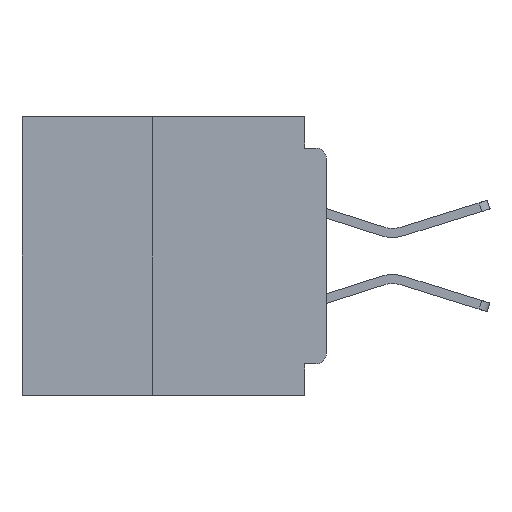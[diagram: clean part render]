
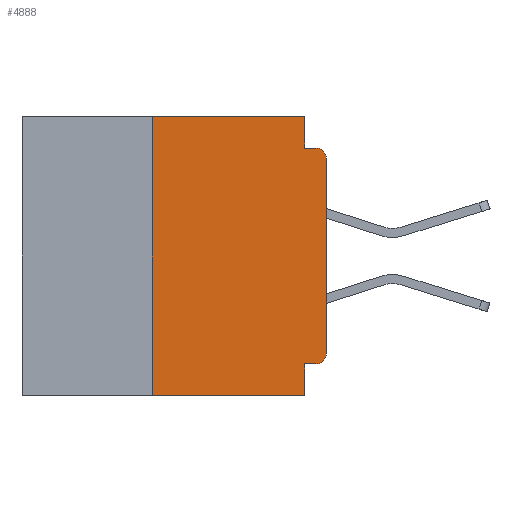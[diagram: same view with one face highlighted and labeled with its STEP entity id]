
A CAD part, left-side view. The second image highlights one B-rep face of the part: STEP entity #4888.
In plain terms, the highlighted planar face has unit normal (-1, 0, 0).
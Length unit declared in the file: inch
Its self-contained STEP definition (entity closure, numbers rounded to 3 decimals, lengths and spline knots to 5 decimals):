
#1334 = ORIENTED_EDGE ( 'NONE', *, *, #21877, .T. ) ;
#1456 = ORIENTED_EDGE ( 'NONE', *, *, #16389, .F. ) ;
#1601 = EDGE_CURVE ( 'NONE', #30420, #3895, #35612, .T. ) ;
#2708 = FACE_OUTER_BOUND ( 'NONE', #19531, .T. ) ;
#3082 = ORIENTED_EDGE ( 'NONE', *, *, #38399, .F. ) ;
#3895 = VERTEX_POINT ( 'NONE', #26321 ) ;
#4888 = ADVANCED_FACE ( 'NONE', ( #2708 ), #45290, .F. ) ;
#5222 = CARTESIAN_POINT ( 'NONE',  ( 0., 0., -0.06 ) ) ;
#5250 = CARTESIAN_POINT ( 'NONE',  ( 0., 0.015, -0.34 ) ) ;
#5289 = EDGE_CURVE ( 'NONE', #10320, #44615, #23680, .T. ) ;
#5556 = VERTEX_POINT ( 'NONE', #16512 ) ;
#5705 = ORIENTED_EDGE ( 'NONE', *, *, #31694, .T. ) ;
#6095 = ORIENTED_EDGE ( 'NONE', *, *, #5289, .F. ) ;
#6575 = CARTESIAN_POINT ( 'NONE',  ( 0., 0.015, -0.355 ) ) ;
#7450 = CARTESIAN_POINT ( 'NONE',  ( 0., 0., -0.045 ) ) ;
#7767 = CARTESIAN_POINT ( 'NONE',  ( 0., 0.25, -0.4 ) ) ;
#8783 = DIRECTION ( 'NONE',  ( 0., 0., -1. ) ) ;
#9641 = VECTOR ( 'NONE', #17980, 39.37008 ) ;
#9995 = LINE ( 'NONE', #41851, #18251 ) ;
#10320 = VERTEX_POINT ( 'NONE', #18087 ) ;
#10326 = DIRECTION ( 'NONE',  ( 0., -1., 0. ) ) ;
#12837 = VECTOR ( 'NONE', #23956, 39.37008 ) ;
#13194 = VERTEX_POINT ( 'NONE', #39578 ) ;
#13732 = EDGE_CURVE ( 'NONE', #3895, #30593, #20109, .T. ) ;
#14413 = CARTESIAN_POINT ( 'NONE',  ( 0., 0.031, -0.4 ) ) ;
#14855 = AXIS2_PLACEMENT_3D ( 'NONE', #44975, #44674, #44639 ) ;
#16389 = EDGE_CURVE ( 'NONE', #18699, #10320, #9995, .T. ) ;
#16512 = CARTESIAN_POINT ( 'NONE',  ( 0., 0.015, -0.045 ) ) ;
#16825 = VECTOR ( 'NONE', #38955, 39.37008 ) ;
#17869 = VERTEX_POINT ( 'NONE', #7767 ) ;
#17980 = DIRECTION ( 'NONE',  ( 0., 0., -1. ) ) ;
#18087 = CARTESIAN_POINT ( 'NONE',  ( 0., 0.031, 0. ) ) ;
#18251 = VECTOR ( 'NONE', #10326, 39.37008 ) ;
#18559 = CIRCLE ( 'NONE', #26442, 0.015 ) ;
#18699 = VERTEX_POINT ( 'NONE', #35764 ) ;
#18898 = EDGE_CURVE ( 'NONE', #30420, #13194, #18559, .T. ) ;
#19531 = EDGE_LOOP ( 'NONE', ( #5705, #1334, #25753, #6095, #1456, #3082, #44940, #28429, #26137, #43435 ) ) ;
#20109 = LINE ( 'NONE', #14413, #9641 ) ;
#20472 = EDGE_CURVE ( 'NONE', #44615, #5556, #40925, .T. ) ;
#20617 = CARTESIAN_POINT ( 'NONE',  ( 0., 0., 0. ) ) ;
#20656 = VECTOR ( 'NONE', #34795, 39.37008 ) ;
#21067 = CARTESIAN_POINT ( 'NONE',  ( 0., 0.015, -0.06 ) ) ;
#21877 = EDGE_CURVE ( 'NONE', #38061, #5556, #42961, .T. ) ;
#22229 = VECTOR ( 'NONE', #38963, 39.37008 ) ;
#23680 = LINE ( 'NONE', #29324, #31943 ) ;
#23802 = LINE ( 'NONE', #45582, #32065 ) ;
#23956 = DIRECTION ( 'NONE',  ( 0., -1., 0. ) ) ;
#24656 = DIRECTION ( 'NONE',  ( 0., 0., -1. ) ) ;
#25753 = ORIENTED_EDGE ( 'NONE', *, *, #20472, .F. ) ;
#26137 = ORIENTED_EDGE ( 'NONE', *, *, #1601, .F. ) ;
#26321 = CARTESIAN_POINT ( 'NONE',  ( 0., 0.031, -0.355 ) ) ;
#26442 = AXIS2_PLACEMENT_3D ( 'NONE', #5250, #29913, #8783 ) ;
#27306 = EDGE_CURVE ( 'NONE', #17869, #30593, #42039, .T. ) ;
#28429 = ORIENTED_EDGE ( 'NONE', *, *, #13732, .F. ) ;
#29119 = DIRECTION ( 'NONE',  ( 0., 0., -1. ) ) ;
#29324 = CARTESIAN_POINT ( 'NONE',  ( 0., 0.031, 0. ) ) ;
#29913 = DIRECTION ( 'NONE',  ( -1., 0., 0. ) ) ;
#30058 = LINE ( 'NONE', #20617, #20656 ) ;
#30420 = VERTEX_POINT ( 'NONE', #6575 ) ;
#30593 = VERTEX_POINT ( 'NONE', #42686 ) ;
#31694 = EDGE_CURVE ( 'NONE', #13194, #38061, #30058, .T. ) ;
#31943 = VECTOR ( 'NONE', #29119, 39.37008 ) ;
#32065 = VECTOR ( 'NONE', #35234, 39.37008 ) ;
#33924 = AXIS2_PLACEMENT_3D ( 'NONE', #21067, #38699, #24656 ) ;
#34795 = DIRECTION ( 'NONE',  ( 0., 0., 1. ) ) ;
#35234 = DIRECTION ( 'NONE',  ( 0., 0., 1. ) ) ;
#35612 = LINE ( 'NONE', #37975, #16825 ) ;
#35764 = CARTESIAN_POINT ( 'NONE',  ( 0., 0.25, 0. ) ) ;
#37930 = CARTESIAN_POINT ( 'NONE',  ( 0., 0.437, -0.4 ) ) ;
#37975 = CARTESIAN_POINT ( 'NONE',  ( 0., 0., -0.355 ) ) ;
#38061 = VERTEX_POINT ( 'NONE', #5222 ) ;
#38399 = EDGE_CURVE ( 'NONE', #17869, #18699, #23802, .T. ) ;
#38699 = DIRECTION ( 'NONE',  ( -1., 0., 0. ) ) ;
#38955 = DIRECTION ( 'NONE',  ( 0., 1., 0. ) ) ;
#38963 = DIRECTION ( 'NONE',  ( 0., -1., 0. ) ) ;
#39578 = CARTESIAN_POINT ( 'NONE',  ( 0., 0., -0.34 ) ) ;
#40925 = LINE ( 'NONE', #7450, #22229 ) ;
#41851 = CARTESIAN_POINT ( 'NONE',  ( 0., 0.437, 0. ) ) ;
#42039 = LINE ( 'NONE', #37930, #12837 ) ;
#42686 = CARTESIAN_POINT ( 'NONE',  ( 0., 0.031, -0.4 ) ) ;
#42961 = CIRCLE ( 'NONE', #33924, 0.015 ) ;
#43435 = ORIENTED_EDGE ( 'NONE', *, *, #18898, .T. ) ;
#43680 = CARTESIAN_POINT ( 'NONE',  ( 0., 0.031, -0.045 ) ) ;
#44615 = VERTEX_POINT ( 'NONE', #43680 ) ;
#44639 = DIRECTION ( 'NONE',  ( 0., 0., -1. ) ) ;
#44674 = DIRECTION ( 'NONE',  ( 1., 0., 0. ) ) ;
#44940 = ORIENTED_EDGE ( 'NONE', *, *, #27306, .T. ) ;
#44975 = CARTESIAN_POINT ( 'NONE',  ( 0., 0.437, 0. ) ) ;
#45290 = PLANE ( 'NONE',  #14855 ) ;
#45582 = CARTESIAN_POINT ( 'NONE',  ( 0., 0.25, -0.4 ) ) ;
